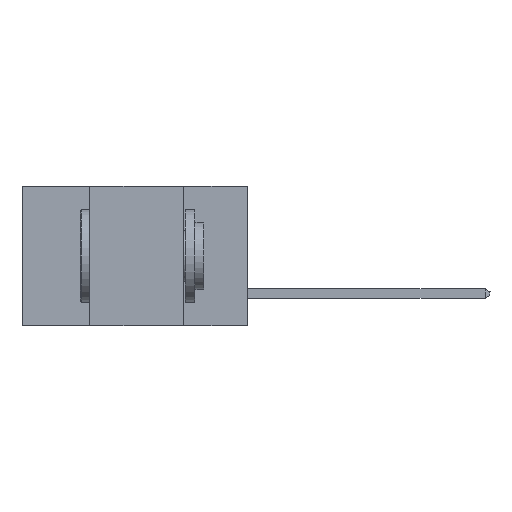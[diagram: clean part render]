
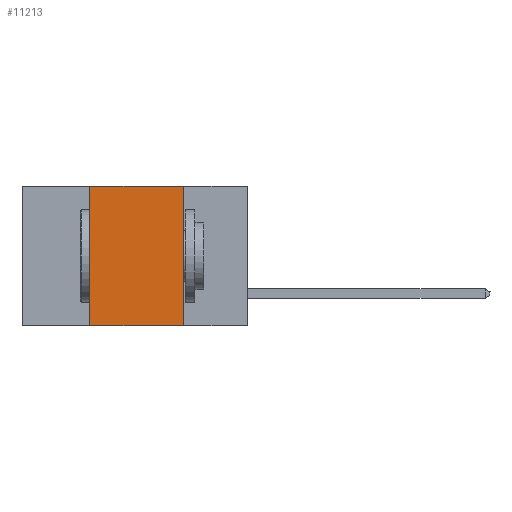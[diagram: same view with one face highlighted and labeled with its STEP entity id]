
A CAD part, left-side view. The second image highlights one B-rep face of the part: STEP entity #11213.
In plain terms, the highlighted planar face has unit normal (-1, 0, 0).
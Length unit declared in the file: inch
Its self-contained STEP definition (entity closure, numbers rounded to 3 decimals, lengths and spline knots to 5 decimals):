
#234 = LINE ( 'NONE', #8951, #6296 ) ;
#595 = DIRECTION ( 'NONE',  ( 0., 0., -1. ) ) ;
#2181 = VERTEX_POINT ( 'NONE', #20380 ) ;
#4322 = PLANE ( 'NONE',  #8768 ) ;
#5868 = EDGE_CURVE ( 'NONE', #21179, #2181, #20698, .T. ) ;
#6180 = FACE_OUTER_BOUND ( 'NONE', #21762, .T. ) ;
#6296 = VECTOR ( 'NONE', #16117, 39.37008 ) ;
#6975 = EDGE_CURVE ( 'NONE', #9743, #2181, #14629, .T. ) ;
#7793 = VECTOR ( 'NONE', #13642, 39.37008 ) ;
#8258 = CARTESIAN_POINT ( 'NONE',  ( 0., 0.6, -0.37 ) ) ;
#8768 = AXIS2_PLACEMENT_3D ( 'NONE', #9325, #21782, #595 ) ;
#8951 = CARTESIAN_POINT ( 'NONE',  ( 0., 0.42, -0.37 ) ) ;
#8965 = CARTESIAN_POINT ( 'NONE',  ( 0., 0.17, 0. ) ) ;
#9219 = ORIENTED_EDGE ( 'NONE', *, *, #12449, .F. ) ;
#9325 = CARTESIAN_POINT ( 'NONE',  ( 0., 0.6, 0. ) ) ;
#9743 = VERTEX_POINT ( 'NONE', #8965 ) ;
#10467 = VECTOR ( 'NONE', #10894, 39.37008 ) ;
#10781 = CARTESIAN_POINT ( 'NONE',  ( 0., 0.6, 0. ) ) ;
#10894 = DIRECTION ( 'NONE',  ( 0., 0., -1. ) ) ;
#11213 = ADVANCED_FACE ( 'NONE', ( #6180 ), #4322, .F. ) ;
#12449 = EDGE_CURVE ( 'NONE', #21179, #18454, #234, .T. ) ;
#13642 = DIRECTION ( 'NONE',  ( 0., -1., 0. ) ) ;
#13833 = VECTOR ( 'NONE', #19795, 39.37008 ) ;
#14629 = LINE ( 'NONE', #16618, #10467 ) ;
#15539 = ORIENTED_EDGE ( 'NONE', *, *, #6975, .F. ) ;
#15756 = CARTESIAN_POINT ( 'NONE',  ( 0., 0.42, 0. ) ) ;
#16117 = DIRECTION ( 'NONE',  ( 0., 0., 1. ) ) ;
#16618 = CARTESIAN_POINT ( 'NONE',  ( 0., 0.17, -0.37 ) ) ;
#18219 = EDGE_CURVE ( 'NONE', #18454, #9743, #19561, .T. ) ;
#18454 = VERTEX_POINT ( 'NONE', #15756 ) ;
#19561 = LINE ( 'NONE', #10781, #13833 ) ;
#19614 = ORIENTED_EDGE ( 'NONE', *, *, #5868, .T. ) ;
#19795 = DIRECTION ( 'NONE',  ( 0., -1., 0. ) ) ;
#20380 = CARTESIAN_POINT ( 'NONE',  ( 0., 0.17, -0.37 ) ) ;
#20698 = LINE ( 'NONE', #8258, #7793 ) ;
#21179 = VERTEX_POINT ( 'NONE', #22276 ) ;
#21762 = EDGE_LOOP ( 'NONE', ( #15539, #22980, #9219, #19614 ) ) ;
#21782 = DIRECTION ( 'NONE',  ( 1., 0., 0. ) ) ;
#22276 = CARTESIAN_POINT ( 'NONE',  ( 0., 0.42, -0.37 ) ) ;
#22980 = ORIENTED_EDGE ( 'NONE', *, *, #18219, .F. ) ;
